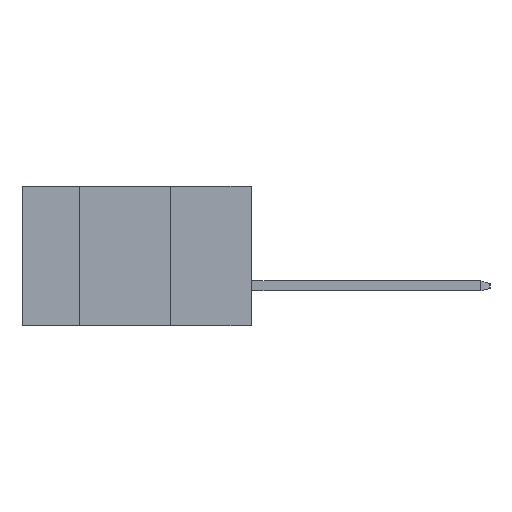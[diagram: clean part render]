
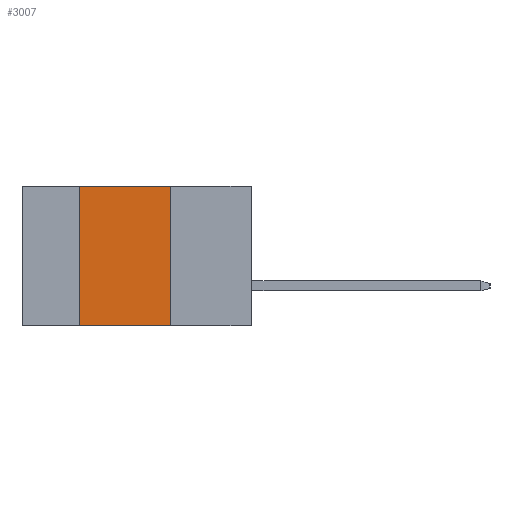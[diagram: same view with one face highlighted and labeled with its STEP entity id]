
A CAD part, left-side view. The second image highlights one B-rep face of the part: STEP entity #3007.
In plain terms, the highlighted planar face has unit normal (-1, 0, 0).
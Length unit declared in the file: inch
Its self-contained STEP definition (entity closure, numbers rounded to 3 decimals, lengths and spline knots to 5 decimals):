
#2 = VECTOR ( 'NONE', #8408, 39.37008 ) ;
#37 = AXIS2_PLACEMENT_3D ( 'NONE', #5360, #325, #9585 ) ;
#74 = VECTOR ( 'NONE', #8806, 39.37008 ) ;
#213 = CARTESIAN_POINT ( 'NONE',  ( 0., 0.54, -0.437 ) ) ;
#325 = DIRECTION ( 'NONE',  ( 1., 0., 0. ) ) ;
#408 = EDGE_CURVE ( 'NONE', #7772, #7310, #7880, .T. ) ;
#425 = LINE ( 'NONE', #10447, #9365 ) ;
#819 = CARTESIAN_POINT ( 'NONE',  ( 0., 0.54, -0.437 ) ) ;
#830 = CARTESIAN_POINT ( 'NONE',  ( 0., 0.254, -0.437 ) ) ;
#1221 = ORIENTED_EDGE ( 'NONE', *, *, #408, .F. ) ;
#1263 = CARTESIAN_POINT ( 'NONE',  ( 0., 0.254, -0.437 ) ) ;
#1388 = EDGE_LOOP ( 'NONE', ( #7674, #1221, #2489, #8221 ) ) ;
#1868 = LINE ( 'NONE', #819, #10625 ) ;
#1970 = EDGE_CURVE ( 'NONE', #7310, #5174, #10194, .T. ) ;
#2489 = ORIENTED_EDGE ( 'NONE', *, *, #9957, .F. ) ;
#2577 = DIRECTION ( 'NONE',  ( 0., 0., 1. ) ) ;
#2846 = DIRECTION ( 'NONE',  ( 0., -1., 0. ) ) ;
#3000 = CARTESIAN_POINT ( 'NONE',  ( 0., 0.72, 0. ) ) ;
#3007 = ADVANCED_FACE ( 'NONE', ( #4384 ), #10173, .F. ) ;
#3744 = CARTESIAN_POINT ( 'NONE',  ( 0., 0.254, 0. ) ) ;
#4384 = FACE_OUTER_BOUND ( 'NONE', #1388, .T. ) ;
#5174 = VERTEX_POINT ( 'NONE', #1263 ) ;
#5360 = CARTESIAN_POINT ( 'NONE',  ( 0., 0.72, 0. ) ) ;
#5473 = CARTESIAN_POINT ( 'NONE',  ( 0., 0.54, 0. ) ) ;
#6173 = VERTEX_POINT ( 'NONE', #213 ) ;
#7310 = VERTEX_POINT ( 'NONE', #3744 ) ;
#7674 = ORIENTED_EDGE ( 'NONE', *, *, #1970, .F. ) ;
#7772 = VERTEX_POINT ( 'NONE', #5473 ) ;
#7880 = LINE ( 'NONE', #3000, #74 ) ;
#8221 = ORIENTED_EDGE ( 'NONE', *, *, #9308, .T. ) ;
#8408 = DIRECTION ( 'NONE',  ( 0., 0., -1. ) ) ;
#8806 = DIRECTION ( 'NONE',  ( 0., -1., 0. ) ) ;
#9308 = EDGE_CURVE ( 'NONE', #6173, #5174, #425, .T. ) ;
#9365 = VECTOR ( 'NONE', #2846, 39.37008 ) ;
#9585 = DIRECTION ( 'NONE',  ( 0., 0., -1. ) ) ;
#9957 = EDGE_CURVE ( 'NONE', #6173, #7772, #1868, .T. ) ;
#10173 = PLANE ( 'NONE',  #37 ) ;
#10194 = LINE ( 'NONE', #830, #2 ) ;
#10447 = CARTESIAN_POINT ( 'NONE',  ( 0., 0.72, -0.437 ) ) ;
#10625 = VECTOR ( 'NONE', #2577, 39.37008 ) ;
